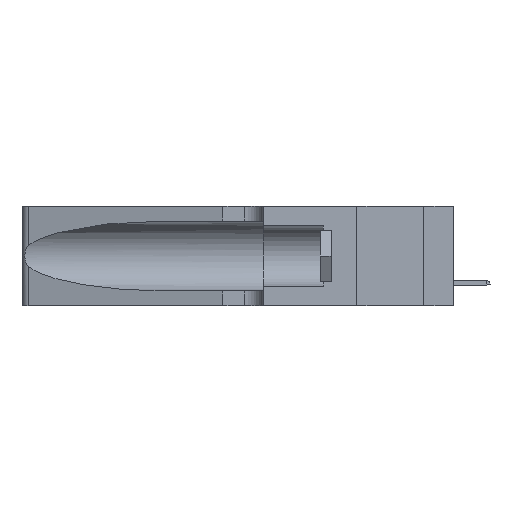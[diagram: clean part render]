
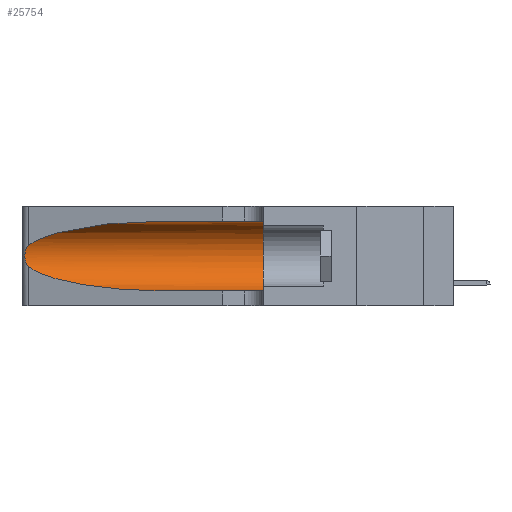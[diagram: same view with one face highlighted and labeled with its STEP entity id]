
A CAD part, left-side view. The second image highlights one B-rep face of the part: STEP entity #25754.
In plain terms, the highlighted cylindrical face has radius 3.308 mm (diameter 6.617 mm), a partial arc.
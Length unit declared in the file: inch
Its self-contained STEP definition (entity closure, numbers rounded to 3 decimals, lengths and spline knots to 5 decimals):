
#393 = EDGE_CURVE ( 'NONE', #29666, #8604, #11657, .T. ) ;
#846 = CARTESIAN_POINT ( 'NONE',  ( 0.1305, 0.72297, 0.31525 ) ) ;
#938 = AXIS2_PLACEMENT_3D ( 'NONE', #6444, #22832, #16377 ) ;
#1059 = CARTESIAN_POINT ( 'NONE',  ( 0.25487, 1.22718, 0.14631 ) ) ;
#2404 = VECTOR ( 'NONE', #21213, 39.37008 ) ;
#3024 = CARTESIAN_POINT ( 'NONE',  ( 0.26075, 1.23896, 0.19203 ) ) ;
#3175 = CARTESIAN_POINT ( 'NONE',  ( 0.26018, 1.23835, 0.19895 ) ) ;
#3618 = VERTEX_POINT ( 'NONE', #27458 ) ;
#4253 = CARTESIAN_POINT ( 'NONE',  ( 0.2373, 1.15595, 0.08982 ) ) ;
#5267 = CARTESIAN_POINT ( 'NONE',  ( 0.25487, 1.22718, 0.22369 ) ) ;
#5865 = AXIS2_PLACEMENT_3D ( 'NONE', #29415, #27412, #26957 ) ;
#6261 = CYLINDRICAL_SURFACE ( 'NONE', #5865, 0.13025 ) ;
#6444 = CARTESIAN_POINT ( 'NONE',  ( 0.1305, 0.35, 0.185 ) ) ;
#8604 = VERTEX_POINT ( 'NONE', #22429 ) ;
#9375 = DIRECTION ( 'NONE',  ( 0., -1., 0. ) ) ;
#9575 = ORIENTED_EDGE ( 'NONE', *, *, #17828, .T. ) ;
#9690 = VERTEX_POINT ( 'NONE', #25166 ) ;
#10370 = CARTESIAN_POINT ( 'NONE',  ( 0.25854, 1.2359, 0.20912 ) ) ;
#11657 = LINE ( 'NONE', #21027, #25029 ) ;
#11856 = LINE ( 'NONE', #23231, #2404 ) ;
#12768 = CARTESIAN_POINT ( 'NONE',  ( 0.2373, 1.15595, 0.28018 ) ) ;
#13625 = B_SPLINE_CURVE_WITH_KNOTS ( 'NONE', 3,
 ( #17417, #14812, #23879, #19573, #10370, #3175, #3024, #19877, #21573, #21870, #26774, #24487, #28927, #1059 ),
 .UNSPECIFIED., .F., .F.,
 ( 4, 2, 2, 2, 2, 2, 4 ),
 ( 0., 0.00027, 0.00053, 0.00107, 0.0016, 0.00187, 0.00214 ),
 .UNSPECIFIED. ) ;
#14091 = EDGE_CURVE ( 'NONE', #17358, #3618, #11856, .T. ) ;
#14747 = EDGE_LOOP ( 'NONE', ( #9575, #18539, #29696, #22152, #24307, #29627 ) ) ;
#14812 = CARTESIAN_POINT ( 'NONE',  ( 0.25555, 1.22994, 0.2215 ) ) ;
#15459 =( BOUNDED_CURVE ( )  B_SPLINE_CURVE ( 3, ( #846, #26727, #12768, #5267 ),
 .UNSPECIFIED., .F., .T. ) 
 B_SPLINE_CURVE_WITH_KNOTS ( ( 4, 4 ),
 ( 1.5708, 2.84003 ),
 .UNSPECIFIED. ) 
 CURVE ( )  GEOMETRIC_REPRESENTATION_ITEM ( )  RATIONAL_B_SPLINE_CURVE ( ( 1., 0.87, 0.87, 1. ) ) 
 REPRESENTATION_ITEM ( '' )  );
#15905 = CARTESIAN_POINT ( 'NONE',  ( 0.25487, 1.22718, 0.14631 ) ) ;
#16377 = DIRECTION ( 'NONE',  ( 0., 0., 1. ) ) ;
#16674 = EDGE_CURVE ( 'NONE', #9690, #17358, #18408, .T. ) ;
#17358 = VERTEX_POINT ( 'NONE', #19561 ) ;
#17417 = CARTESIAN_POINT ( 'NONE',  ( 0.25487, 1.22718, 0.22369 ) ) ;
#17828 = EDGE_CURVE ( 'NONE', #29666, #24687, #15459, .T. ) ;
#18062 = CIRCLE ( 'NONE', #938, 0.13025 ) ;
#18408 =( BOUNDED_CURVE ( )  B_SPLINE_CURVE ( 3, ( #15905, #4253, #26725, #21966 ),
 .UNSPECIFIED., .F., .T. ) 
 B_SPLINE_CURVE_WITH_KNOTS ( ( 4, 4 ),
 ( 3.44316, 4.71239 ),
 .UNSPECIFIED. ) 
 CURVE ( )  GEOMETRIC_REPRESENTATION_ITEM ( )  RATIONAL_B_SPLINE_CURVE ( ( 1., 0.87, 0.87, 1. ) ) 
 REPRESENTATION_ITEM ( '' )  );
#18539 = ORIENTED_EDGE ( 'NONE', *, *, #27485, .T. ) ;
#19561 = CARTESIAN_POINT ( 'NONE',  ( 0.1305, 0.72297, 0.05475 ) ) ;
#19573 = CARTESIAN_POINT ( 'NONE',  ( 0.25787, 1.23484, 0.2124 ) ) ;
#19877 = CARTESIAN_POINT ( 'NONE',  ( 0.26075, 1.23896, 0.178 ) ) ;
#20671 = FACE_OUTER_BOUND ( 'NONE', #14747, .T. ) ;
#21027 = CARTESIAN_POINT ( 'NONE',  ( 0.1305, 1.61858, 0.31525 ) ) ;
#21213 = DIRECTION ( 'NONE',  ( 0., -1., 0. ) ) ;
#21464 = CARTESIAN_POINT ( 'NONE',  ( 0.25487, 1.22718, 0.22369 ) ) ;
#21573 = CARTESIAN_POINT ( 'NONE',  ( 0.26017, 1.23833, 0.17102 ) ) ;
#21870 = CARTESIAN_POINT ( 'NONE',  ( 0.25856, 1.23593, 0.16098 ) ) ;
#21966 = CARTESIAN_POINT ( 'NONE',  ( 0.1305, 0.72297, 0.05475 ) ) ;
#22152 = ORIENTED_EDGE ( 'NONE', *, *, #14091, .T. ) ;
#22429 = CARTESIAN_POINT ( 'NONE',  ( 0.1305, 0.35, 0.31525 ) ) ;
#22832 = DIRECTION ( 'NONE',  ( 0., 1., 0. ) ) ;
#23231 = CARTESIAN_POINT ( 'NONE',  ( 0.1305, 1.61858, 0.05475 ) ) ;
#23879 = CARTESIAN_POINT ( 'NONE',  ( 0.25639, 1.23184, 0.21858 ) ) ;
#23962 = CARTESIAN_POINT ( 'NONE',  ( 0.1305, 0.72297, 0.31525 ) ) ;
#24307 = ORIENTED_EDGE ( 'NONE', *, *, #24959, .F. ) ;
#24487 = CARTESIAN_POINT ( 'NONE',  ( 0.25639, 1.23186, 0.15144 ) ) ;
#24687 = VERTEX_POINT ( 'NONE', #21464 ) ;
#24959 = EDGE_CURVE ( 'NONE', #8604, #3618, #18062, .T. ) ;
#25029 = VECTOR ( 'NONE', #9375, 39.37008 ) ;
#25166 = CARTESIAN_POINT ( 'NONE',  ( 0.25487, 1.22718, 0.14631 ) ) ;
#25754 = ADVANCED_FACE ( 'NONE', ( #20671 ), #6261, .F. ) ;
#26725 = CARTESIAN_POINT ( 'NONE',  ( 0.18966, 0.96281, 0.05475 ) ) ;
#26727 = CARTESIAN_POINT ( 'NONE',  ( 0.18966, 0.96281, 0.31525 ) ) ;
#26774 = CARTESIAN_POINT ( 'NONE',  ( 0.25789, 1.23486, 0.15765 ) ) ;
#26957 = DIRECTION ( 'NONE',  ( 0., 0., -1. ) ) ;
#27412 = DIRECTION ( 'NONE',  ( 0., -1., 0. ) ) ;
#27458 = CARTESIAN_POINT ( 'NONE',  ( 0.1305, 0.35, 0.05475 ) ) ;
#27485 = EDGE_CURVE ( 'NONE', #24687, #9690, #13625, .T. ) ;
#28927 = CARTESIAN_POINT ( 'NONE',  ( 0.25555, 1.22993, 0.14849 ) ) ;
#29415 = CARTESIAN_POINT ( 'NONE',  ( 0.1305, 1.61858, 0.185 ) ) ;
#29627 = ORIENTED_EDGE ( 'NONE', *, *, #393, .F. ) ;
#29666 = VERTEX_POINT ( 'NONE', #23962 ) ;
#29696 = ORIENTED_EDGE ( 'NONE', *, *, #16674, .T. ) ;
